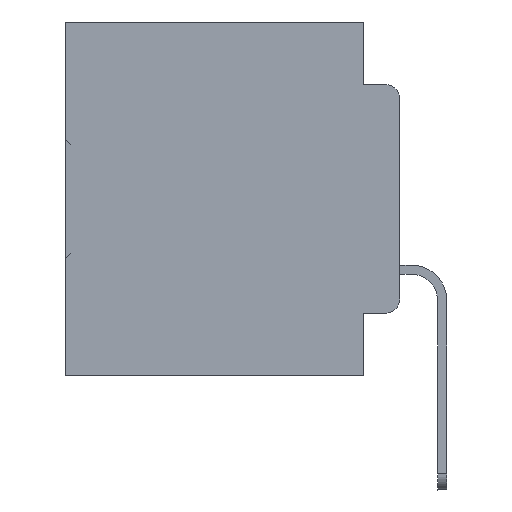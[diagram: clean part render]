
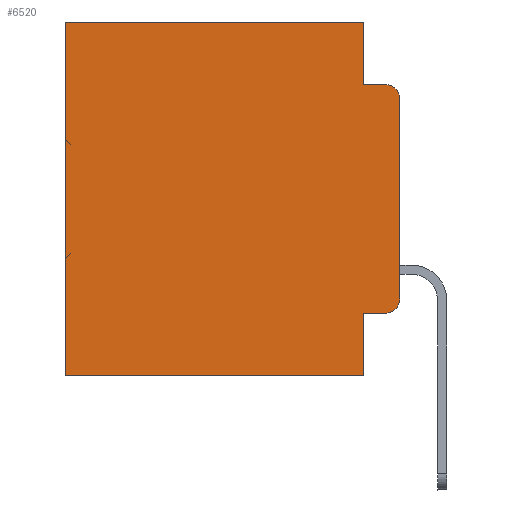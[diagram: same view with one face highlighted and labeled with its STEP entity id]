
A CAD part, left-side view. The second image highlights one B-rep face of the part: STEP entity #6520.
In plain terms, the highlighted planar face has unit normal (-1, 0, 0).
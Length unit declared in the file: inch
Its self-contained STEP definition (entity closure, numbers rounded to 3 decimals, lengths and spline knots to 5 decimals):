
#489 = LINE ( 'NONE', #34028, #28064 ) ;
#1703 = DIRECTION ( 'NONE',  ( 0., 0., -1. ) ) ;
#1850 = ORIENTED_EDGE ( 'NONE', *, *, #2364, .F. ) ;
#2056 = CARTESIAN_POINT ( 'NONE',  ( 0.298, 0.02, -0.3915 ) ) ;
#2364 = EDGE_CURVE ( 'NONE', #31820, #4902, #21229, .T. ) ;
#2603 = DIRECTION ( 'NONE',  ( 0., 0., -1. ) ) ;
#2979 = EDGE_CURVE ( 'NONE', #4902, #17788, #30060, .T. ) ;
#3358 = DIRECTION ( 'NONE',  ( -1., 0., 0. ) ) ;
#3964 = VECTOR ( 'NONE', #12159, 39.37008 ) ;
#4177 = CARTESIAN_POINT ( 'NONE',  ( 0.298, 0., -0.1085 ) ) ;
#4370 = CARTESIAN_POINT ( 'NONE',  ( 0.298, 0.051, 0. ) ) ;
#4902 = VERTEX_POINT ( 'NONE', #26360 ) ;
#5484 = CARTESIAN_POINT ( 'NONE',  ( 0.298, 0., -0.3915 ) ) ;
#5850 = CARTESIAN_POINT ( 'NONE',  ( 0.298, 0., -0.5 ) ) ;
#6520 = ADVANCED_FACE ( 'NONE', ( #23651 ), #17856, .F. ) ;
#6532 = VERTEX_POINT ( 'NONE', #8566 ) ;
#7862 = LINE ( 'NONE', #33229, #18772 ) ;
#8308 = VERTEX_POINT ( 'NONE', #5484 ) ;
#8566 = CARTESIAN_POINT ( 'NONE',  ( 0.298, 0.02, -0.4115 ) ) ;
#8660 = ORIENTED_EDGE ( 'NONE', *, *, #16375, .T. ) ;
#8718 = DIRECTION ( 'NONE',  ( 0., 1., 0. ) ) ;
#11348 = DIRECTION ( 'NONE',  ( 0., 0., -1. ) ) ;
#12159 = DIRECTION ( 'NONE',  ( 0., -1., 0. ) ) ;
#12289 = EDGE_CURVE ( 'NONE', #16532, #17788, #18742, .T. ) ;
#12704 = LINE ( 'NONE', #25940, #3964 ) ;
#13251 = ORIENTED_EDGE ( 'NONE', *, *, #25356, .F. ) ;
#14048 = EDGE_CURVE ( 'NONE', #26568, #22121, #30695, .T. ) ;
#14124 = AXIS2_PLACEMENT_3D ( 'NONE', #23080, #3358, #20355 ) ;
#14140 = ORIENTED_EDGE ( 'NONE', *, *, #31528, .T. ) ;
#15055 = VECTOR ( 'NONE', #18674, 39.37008 ) ;
#15131 = DIRECTION ( 'NONE',  ( 1., 0., 0. ) ) ;
#15611 = VERTEX_POINT ( 'NONE', #20020 ) ;
#16375 = EDGE_CURVE ( 'NONE', #31820, #18839, #30489, .T. ) ;
#16532 = VERTEX_POINT ( 'NONE', #4177 ) ;
#17398 = CARTESIAN_POINT ( 'NONE',  ( 0.298, 0.02, -0.0885 ) ) ;
#17788 = VERTEX_POINT ( 'NONE', #17398 ) ;
#17856 = PLANE ( 'NONE',  #27388 ) ;
#18147 = AXIS2_PLACEMENT_3D ( 'NONE', #2056, #18882, #1703 ) ;
#18193 = CARTESIAN_POINT ( 'NONE',  ( 0.298, 0.473, -0.5 ) ) ;
#18674 = DIRECTION ( 'NONE',  ( 0., 0., -1. ) ) ;
#18742 = CIRCLE ( 'NONE', #14124, 0.02 ) ;
#18772 = VECTOR ( 'NONE', #2603, 39.37008 ) ;
#18839 = VERTEX_POINT ( 'NONE', #21305 ) ;
#18842 = VECTOR ( 'NONE', #19784, 39.37008 ) ;
#18882 = DIRECTION ( 'NONE',  ( -1., 0., 0. ) ) ;
#19166 = CARTESIAN_POINT ( 'NONE',  ( 0.298, 0.051, -0.0885 ) ) ;
#19610 = EDGE_CURVE ( 'NONE', #15611, #6532, #12704, .T. ) ;
#19784 = DIRECTION ( 'NONE',  ( 0., 1., 0. ) ) ;
#20020 = CARTESIAN_POINT ( 'NONE',  ( 0.298, 0.051, -0.4115 ) ) ;
#20355 = DIRECTION ( 'NONE',  ( 0., 0., -1. ) ) ;
#21098 = VECTOR ( 'NONE', #29100, 39.37008 ) ;
#21229 = LINE ( 'NONE', #35381, #15055 ) ;
#21305 = CARTESIAN_POINT ( 'NONE',  ( 0.298, 0.473, 0. ) ) ;
#21791 = LINE ( 'NONE', #30124, #21098 ) ;
#21918 = ORIENTED_EDGE ( 'NONE', *, *, #14048, .F. ) ;
#22017 = VECTOR ( 'NONE', #30241, 39.37008 ) ;
#22121 = VERTEX_POINT ( 'NONE', #18193 ) ;
#23080 = CARTESIAN_POINT ( 'NONE',  ( 0.298, 0.02, -0.1085 ) ) ;
#23651 = FACE_OUTER_BOUND ( 'NONE', #32241, .T. ) ;
#24764 = ORIENTED_EDGE ( 'NONE', *, *, #32428, .T. ) ;
#25356 = EDGE_CURVE ( 'NONE', #16532, #8308, #489, .T. ) ;
#25940 = CARTESIAN_POINT ( 'NONE',  ( 0.298, 0.051, -0.4115 ) ) ;
#26185 = DIRECTION ( 'NONE',  ( 0., 0., -1. ) ) ;
#26360 = CARTESIAN_POINT ( 'NONE',  ( 0.298, 0.051, -0.0885 ) ) ;
#26568 = VERTEX_POINT ( 'NONE', #26633 ) ;
#26633 = CARTESIAN_POINT ( 'NONE',  ( 0.298, 0.051, -0.5 ) ) ;
#27199 = ORIENTED_EDGE ( 'NONE', *, *, #34228, .F. ) ;
#27388 = AXIS2_PLACEMENT_3D ( 'NONE', #28910, #15131, #26185 ) ;
#27686 = ORIENTED_EDGE ( 'NONE', *, *, #12289, .T. ) ;
#28064 = VECTOR ( 'NONE', #11348, 39.37008 ) ;
#28910 = CARTESIAN_POINT ( 'NONE',  ( 0.298, 0., 0. ) ) ;
#29100 = DIRECTION ( 'NONE',  ( 0., 0., -1. ) ) ;
#29500 = ORIENTED_EDGE ( 'NONE', *, *, #2979, .F. ) ;
#30060 = LINE ( 'NONE', #19166, #22017 ) ;
#30124 = CARTESIAN_POINT ( 'NONE',  ( 0.298, 0.473, 0. ) ) ;
#30241 = DIRECTION ( 'NONE',  ( 0., -1., 0. ) ) ;
#30489 = LINE ( 'NONE', #30659, #32828 ) ;
#30659 = CARTESIAN_POINT ( 'NONE',  ( 0.298, 0., 0. ) ) ;
#30695 = LINE ( 'NONE', #5850, #18842 ) ;
#31528 = EDGE_CURVE ( 'NONE', #6532, #8308, #33802, .T. ) ;
#31820 = VERTEX_POINT ( 'NONE', #4370 ) ;
#32241 = EDGE_LOOP ( 'NONE', ( #13251, #27686, #29500, #1850, #8660, #24764, #21918, #27199, #33930, #14140 ) ) ;
#32428 = EDGE_CURVE ( 'NONE', #18839, #22121, #21791, .T. ) ;
#32828 = VECTOR ( 'NONE', #8718, 39.37008 ) ;
#33229 = CARTESIAN_POINT ( 'NONE',  ( 0.298, 0.051, 0. ) ) ;
#33802 = CIRCLE ( 'NONE', #18147, 0.02 ) ;
#33930 = ORIENTED_EDGE ( 'NONE', *, *, #19610, .T. ) ;
#34028 = CARTESIAN_POINT ( 'NONE',  ( 0.298, 0., 0. ) ) ;
#34228 = EDGE_CURVE ( 'NONE', #15611, #26568, #7862, .T. ) ;
#35381 = CARTESIAN_POINT ( 'NONE',  ( 0.298, 0.051, 0. ) ) ;
